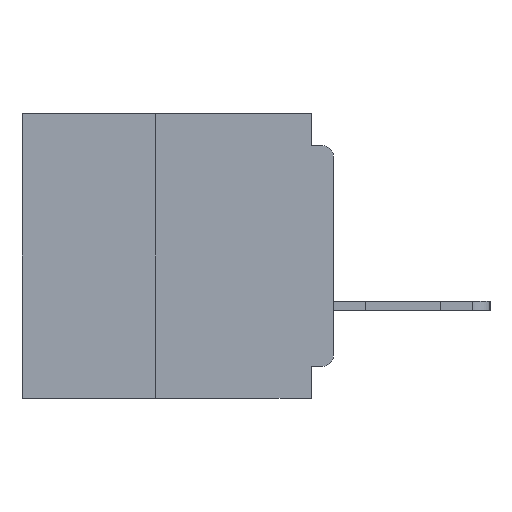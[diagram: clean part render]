
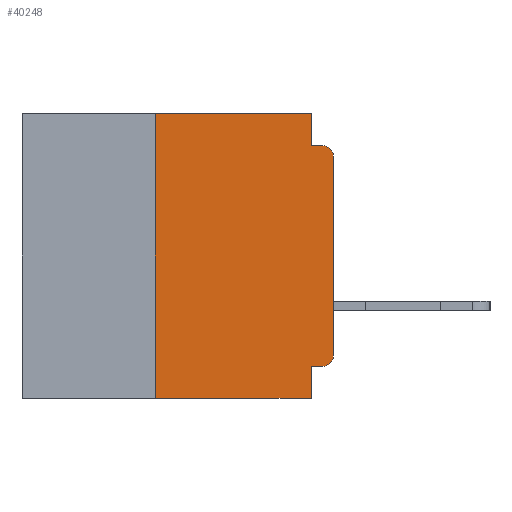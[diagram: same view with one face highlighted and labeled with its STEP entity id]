
A CAD part, left-side view. The second image highlights one B-rep face of the part: STEP entity #40248.
In plain terms, the highlighted planar face has unit normal (-1, 0, 0).
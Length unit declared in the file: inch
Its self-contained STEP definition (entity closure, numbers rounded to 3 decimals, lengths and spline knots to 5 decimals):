
#228 = ORIENTED_EDGE ( 'NONE', *, *, #6852, .T. ) ;
#582 = CARTESIAN_POINT ( 'NONE',  ( 0., 0.015, -0.06 ) ) ;
#1519 = VERTEX_POINT ( 'NONE', #5416 ) ;
#2529 = CIRCLE ( 'NONE', #43049, 0.015 ) ;
#2600 = CARTESIAN_POINT ( 'NONE',  ( 0., 0., -0.34 ) ) ;
#3813 = CARTESIAN_POINT ( 'NONE',  ( 0., 0.015, -0.34 ) ) ;
#4296 = DIRECTION ( 'NONE',  ( 0., 0., -1. ) ) ;
#4592 = ORIENTED_EDGE ( 'NONE', *, *, #31046, .F. ) ;
#5416 = CARTESIAN_POINT ( 'NONE',  ( 0., 0.015, -0.045 ) ) ;
#6852 = EDGE_CURVE ( 'NONE', #27871, #25167, #29313, .T. ) ;
#7197 = ORIENTED_EDGE ( 'NONE', *, *, #37931, .T. ) ;
#7544 = DIRECTION ( 'NONE',  ( 0., 0., -1. ) ) ;
#9827 = CARTESIAN_POINT ( 'NONE',  ( 0., 0.437, 0. ) ) ;
#9878 = CARTESIAN_POINT ( 'NONE',  ( 0., 0., -0.045 ) ) ;
#9911 = DIRECTION ( 'NONE',  ( 0., 0., -1. ) ) ;
#10030 = VECTOR ( 'NONE', #35688, 39.37008 ) ;
#10740 = CARTESIAN_POINT ( 'NONE',  ( 0., 0.015, -0.355 ) ) ;
#11100 = CARTESIAN_POINT ( 'NONE',  ( 0., 0.25, -0.4 ) ) ;
#11684 = DIRECTION ( 'NONE',  ( 0., 1., 0. ) ) ;
#11752 = ORIENTED_EDGE ( 'NONE', *, *, #13172, .F. ) ;
#12340 = VECTOR ( 'NONE', #37491, 39.37008 ) ;
#12912 = AXIS2_PLACEMENT_3D ( 'NONE', #9827, #17115, #17269 ) ;
#13172 = EDGE_CURVE ( 'NONE', #27436, #25167, #21551, .T. ) ;
#13543 = PLANE ( 'NONE',  #12912 ) ;
#15554 = CARTESIAN_POINT ( 'NONE',  ( 0., 0.25, -0.4 ) ) ;
#15791 = EDGE_CURVE ( 'NONE', #45755, #1519, #20020, .T. ) ;
#17107 = CARTESIAN_POINT ( 'NONE',  ( 0., 0.031, 0. ) ) ;
#17115 = DIRECTION ( 'NONE',  ( 1., 0., 0. ) ) ;
#17269 = DIRECTION ( 'NONE',  ( 0., 0., -1. ) ) ;
#17673 = ORIENTED_EDGE ( 'NONE', *, *, #33049, .F. ) ;
#18291 = CARTESIAN_POINT ( 'NONE',  ( 0., 0.031, -0.045 ) ) ;
#18414 = EDGE_CURVE ( 'NONE', #36004, #41575, #30519, .T. ) ;
#18514 = VECTOR ( 'NONE', #11684, 39.37008 ) ;
#19683 = VECTOR ( 'NONE', #45256, 39.37008 ) ;
#20020 = CIRCLE ( 'NONE', #28613, 0.015 ) ;
#21289 = VECTOR ( 'NONE', #34397, 39.37008 ) ;
#21551 = LINE ( 'NONE', #24592, #39591 ) ;
#22218 = LINE ( 'NONE', #15554, #12340 ) ;
#22429 = LINE ( 'NONE', #30775, #21289 ) ;
#22868 = CARTESIAN_POINT ( 'NONE',  ( 0., 0.031, -0.4 ) ) ;
#23425 = EDGE_CURVE ( 'NONE', #40942, #27436, #37792, .T. ) ;
#24592 = CARTESIAN_POINT ( 'NONE',  ( 0., 0.031, -0.4 ) ) ;
#24800 = EDGE_CURVE ( 'NONE', #28944, #45755, #22429, .T. ) ;
#25167 = VERTEX_POINT ( 'NONE', #22868 ) ;
#26302 = CARTESIAN_POINT ( 'NONE',  ( 0., 0., -0.355 ) ) ;
#26378 = DIRECTION ( 'NONE',  ( -1., 0., 0. ) ) ;
#27436 = VERTEX_POINT ( 'NONE', #30525 ) ;
#27577 = VECTOR ( 'NONE', #46451, 39.37008 ) ;
#27871 = VERTEX_POINT ( 'NONE', #11100 ) ;
#28205 = CARTESIAN_POINT ( 'NONE',  ( 0., 0.031, 0. ) ) ;
#28206 = DIRECTION ( 'NONE',  ( 0., 0., -1. ) ) ;
#28539 = ORIENTED_EDGE ( 'NONE', *, *, #24800, .T. ) ;
#28613 = AXIS2_PLACEMENT_3D ( 'NONE', #582, #26378, #4296 ) ;
#28944 = VERTEX_POINT ( 'NONE', #2600 ) ;
#29313 = LINE ( 'NONE', #34277, #19683 ) ;
#29380 = VECTOR ( 'NONE', #9911, 39.37008 ) ;
#29548 = DIRECTION ( 'NONE',  ( -1., 0., 0. ) ) ;
#29550 = CARTESIAN_POINT ( 'NONE',  ( 0., 0., -0.06 ) ) ;
#29896 = ORIENTED_EDGE ( 'NONE', *, *, #15791, .T. ) ;
#30519 = LINE ( 'NONE', #28205, #29380 ) ;
#30525 = CARTESIAN_POINT ( 'NONE',  ( 0., 0.031, -0.355 ) ) ;
#30775 = CARTESIAN_POINT ( 'NONE',  ( 0., 0., 0. ) ) ;
#31046 = EDGE_CURVE ( 'NONE', #27871, #47273, #22218, .T. ) ;
#31338 = CARTESIAN_POINT ( 'NONE',  ( 0., 0.25, 0. ) ) ;
#32093 = CARTESIAN_POINT ( 'NONE',  ( 0., 0.437, 0. ) ) ;
#33049 = EDGE_CURVE ( 'NONE', #47273, #36004, #39129, .T. ) ;
#34277 = CARTESIAN_POINT ( 'NONE',  ( 0., 0.437, -0.4 ) ) ;
#34397 = DIRECTION ( 'NONE',  ( 0., 0., 1. ) ) ;
#34989 = EDGE_LOOP ( 'NONE', ( #28539, #29896, #47475, #35984, #17673, #4592, #228, #11752, #38223, #7197 ) ) ;
#35447 = EDGE_CURVE ( 'NONE', #41575, #1519, #37193, .T. ) ;
#35688 = DIRECTION ( 'NONE',  ( 0., -1., 0. ) ) ;
#35984 = ORIENTED_EDGE ( 'NONE', *, *, #18414, .F. ) ;
#36004 = VERTEX_POINT ( 'NONE', #17107 ) ;
#37193 = LINE ( 'NONE', #9878, #27577 ) ;
#37491 = DIRECTION ( 'NONE',  ( 0., 0., 1. ) ) ;
#37792 = LINE ( 'NONE', #26302, #18514 ) ;
#37931 = EDGE_CURVE ( 'NONE', #40942, #28944, #2529, .T. ) ;
#38223 = ORIENTED_EDGE ( 'NONE', *, *, #23425, .F. ) ;
#39121 = FACE_OUTER_BOUND ( 'NONE', #34989, .T. ) ;
#39129 = LINE ( 'NONE', #32093, #10030 ) ;
#39591 = VECTOR ( 'NONE', #28206, 39.37008 ) ;
#40248 = ADVANCED_FACE ( 'NONE', ( #39121 ), #13543, .F. ) ;
#40942 = VERTEX_POINT ( 'NONE', #10740 ) ;
#41575 = VERTEX_POINT ( 'NONE', #18291 ) ;
#43049 = AXIS2_PLACEMENT_3D ( 'NONE', #3813, #29548, #7544 ) ;
#45256 = DIRECTION ( 'NONE',  ( 0., -1., 0. ) ) ;
#45755 = VERTEX_POINT ( 'NONE', #29550 ) ;
#46451 = DIRECTION ( 'NONE',  ( 0., -1., 0. ) ) ;
#47273 = VERTEX_POINT ( 'NONE', #31338 ) ;
#47475 = ORIENTED_EDGE ( 'NONE', *, *, #35447, .F. ) ;
